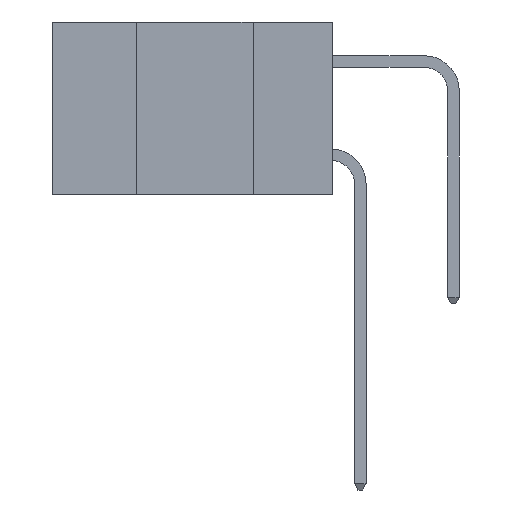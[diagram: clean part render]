
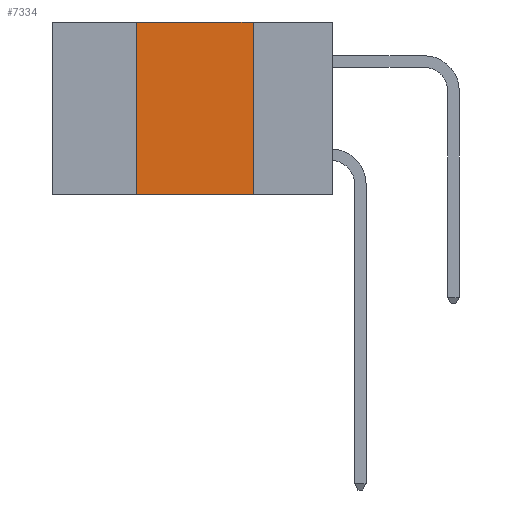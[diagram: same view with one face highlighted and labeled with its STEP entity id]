
A CAD part, left-side view. The second image highlights one B-rep face of the part: STEP entity #7334.
In plain terms, the highlighted planar face has unit normal (-1, 0, 0).
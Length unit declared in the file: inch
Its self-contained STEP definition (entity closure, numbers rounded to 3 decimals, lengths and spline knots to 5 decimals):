
#27 = CARTESIAN_POINT ( 'NONE',  ( 0., 0.17, -0.37 ) ) ;
#181 = LINE ( 'NONE', #3201, #3472 ) ;
#966 = EDGE_CURVE ( 'NONE', #5014, #14911, #11587, .T. ) ;
#1613 = CARTESIAN_POINT ( 'NONE',  ( 0., 0.42, -0.37 ) ) ;
#2155 = CARTESIAN_POINT ( 'NONE',  ( 0., 0.17, 0. ) ) ;
#2792 = VERTEX_POINT ( 'NONE', #1613 ) ;
#2856 = DIRECTION ( 'NONE',  ( 0., -1., 0. ) ) ;
#3201 = CARTESIAN_POINT ( 'NONE',  ( 0., 0.17, -0.37 ) ) ;
#3392 = AXIS2_PLACEMENT_3D ( 'NONE', #12243, #12205, #12131 ) ;
#3472 = VECTOR ( 'NONE', #3582, 39.37008 ) ;
#3476 = LINE ( 'NONE', #9878, #12384 ) ;
#3582 = DIRECTION ( 'NONE',  ( 0., 0., -1. ) ) ;
#4399 = LINE ( 'NONE', #9096, #7258 ) ;
#4423 = FACE_OUTER_BOUND ( 'NONE', #8552, .T. ) ;
#5014 = VERTEX_POINT ( 'NONE', #13059 ) ;
#6000 = ORIENTED_EDGE ( 'NONE', *, *, #13912, .F. ) ;
#6701 = EDGE_CURVE ( 'NONE', #14911, #7933, #181, .T. ) ;
#7258 = VECTOR ( 'NONE', #8932, 39.37008 ) ;
#7334 = ADVANCED_FACE ( 'NONE', ( #4423 ), #13412, .F. ) ;
#7933 = VERTEX_POINT ( 'NONE', #27 ) ;
#8228 = EDGE_CURVE ( 'NONE', #2792, #7933, #4399, .T. ) ;
#8552 = EDGE_LOOP ( 'NONE', ( #9634, #9276, #6000, #11662 ) ) ;
#8932 = DIRECTION ( 'NONE',  ( 0., -1., 0. ) ) ;
#9096 = CARTESIAN_POINT ( 'NONE',  ( 0., 0.6, -0.37 ) ) ;
#9276 = ORIENTED_EDGE ( 'NONE', *, *, #966, .F. ) ;
#9634 = ORIENTED_EDGE ( 'NONE', *, *, #6701, .F. ) ;
#9878 = CARTESIAN_POINT ( 'NONE',  ( 0., 0.42, -0.37 ) ) ;
#9887 = DIRECTION ( 'NONE',  ( 0., 0., 1. ) ) ;
#10840 = VECTOR ( 'NONE', #2856, 39.37008 ) ;
#11587 = LINE ( 'NONE', #12159, #10840 ) ;
#11662 = ORIENTED_EDGE ( 'NONE', *, *, #8228, .T. ) ;
#12131 = DIRECTION ( 'NONE',  ( 0., 0., -1. ) ) ;
#12159 = CARTESIAN_POINT ( 'NONE',  ( 0., 0.6, 0. ) ) ;
#12205 = DIRECTION ( 'NONE',  ( 1., 0., 0. ) ) ;
#12243 = CARTESIAN_POINT ( 'NONE',  ( 0., 0.6, 0. ) ) ;
#12384 = VECTOR ( 'NONE', #9887, 39.37008 ) ;
#13059 = CARTESIAN_POINT ( 'NONE',  ( 0., 0.42, 0. ) ) ;
#13412 = PLANE ( 'NONE',  #3392 ) ;
#13912 = EDGE_CURVE ( 'NONE', #2792, #5014, #3476, .T. ) ;
#14911 = VERTEX_POINT ( 'NONE', #2155 ) ;
